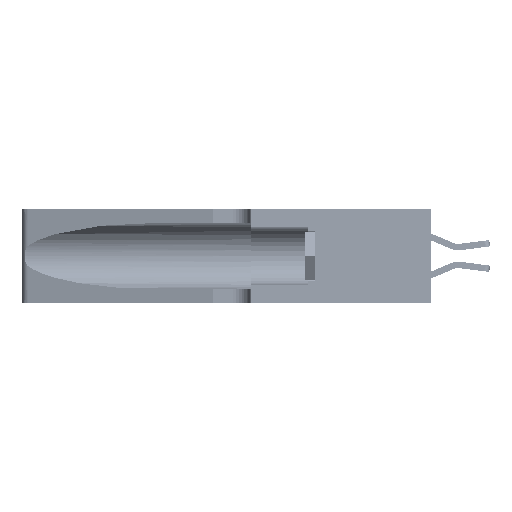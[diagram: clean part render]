
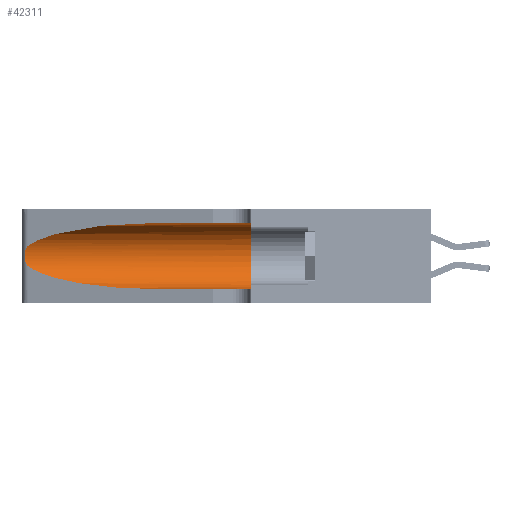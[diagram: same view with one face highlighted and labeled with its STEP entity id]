
A CAD part, left-side view. The second image highlights one B-rep face of the part: STEP entity #42311.
In plain terms, the highlighted cylindrical face has radius 3.308 mm (diameter 6.617 mm), a partial arc.
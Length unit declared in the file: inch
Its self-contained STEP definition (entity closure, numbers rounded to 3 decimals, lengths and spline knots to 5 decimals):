
#1791 = B_SPLINE_CURVE_WITH_KNOTS ( 'NONE', 3,
 ( #13094, #17264, #5121, #40816, #17089, #44774, #29031, #45111, #5292, #5470, #9422, #37172, #38352, #14465 ),
 .UNSPECIFIED., .F., .F.,
 ( 4, 2, 2, 2, 2, 2, 4 ),
 ( 0., 0.00027, 0.00053, 0.00107, 0.0016, 0.00187, 0.00214 ),
 .UNSPECIFIED. ) ;
#2441 = EDGE_CURVE ( 'NONE', #7598, #33572, #5179, .T. ) ;
#2473 = ORIENTED_EDGE ( 'NONE', *, *, #24177, .T. ) ;
#4819 = CARTESIAN_POINT ( 'NONE',  ( 0.18966, 0.96281, 0.31525 ) ) ;
#4823 = CARTESIAN_POINT ( 'NONE',  ( 0.1305, 0.35, 0.185 ) ) ;
#5121 = CARTESIAN_POINT ( 'NONE',  ( 0.25639, 1.23184, 0.21858 ) ) ;
#5179 = CIRCLE ( 'NONE', #12178, 0.13025 ) ;
#5292 = CARTESIAN_POINT ( 'NONE',  ( 0.26017, 1.23833, 0.17102 ) ) ;
#5470 = CARTESIAN_POINT ( 'NONE',  ( 0.25856, 1.23593, 0.16098 ) ) ;
#7160 = ORIENTED_EDGE ( 'NONE', *, *, #2441, .F. ) ;
#7336 = EDGE_LOOP ( 'NONE', ( #2473, #26420, #42686, #13716, #7160, #28904 ) ) ;
#7598 = VERTEX_POINT ( 'NONE', #31393 ) ;
#7652 = CARTESIAN_POINT ( 'NONE',  ( 0.1305, 0.72297, 0.05475 ) ) ;
#8062 = CARTESIAN_POINT ( 'NONE',  ( 0.25487, 1.22718, 0.14631 ) ) ;
#8088 = CARTESIAN_POINT ( 'NONE',  ( 0.1305, 1.61858, 0.05475 ) ) ;
#9422 = CARTESIAN_POINT ( 'NONE',  ( 0.25789, 1.23486, 0.15765 ) ) ;
#9852 = CARTESIAN_POINT ( 'NONE',  ( 0.1305, 0.35, 0.05475 ) ) ;
#10421 = VECTOR ( 'NONE', #28705, 39.37008 ) ;
#12178 = AXIS2_PLACEMENT_3D ( 'NONE', #4823, #48084, #44299 ) ;
#12336 = CARTESIAN_POINT ( 'NONE',  ( 0.1305, 0.72297, 0.31525 ) ) ;
#12973 = CARTESIAN_POINT ( 'NONE',  ( 0.1305, 0.72297, 0.31525 ) ) ;
#13094 = CARTESIAN_POINT ( 'NONE',  ( 0.25487, 1.22718, 0.22369 ) ) ;
#13452 = CARTESIAN_POINT ( 'NONE',  ( 0.1305, 1.61858, 0.31525 ) ) ;
#13587 = AXIS2_PLACEMENT_3D ( 'NONE', #41550, #18192, #29796 ) ;
#13644 = EDGE_CURVE ( 'NONE', #45733, #33572, #19347, .T. ) ;
#13716 = ORIENTED_EDGE ( 'NONE', *, *, #13644, .T. ) ;
#14093 = CYLINDRICAL_SURFACE ( 'NONE', #13587, 0.13025 ) ;
#14465 = CARTESIAN_POINT ( 'NONE',  ( 0.25487, 1.22718, 0.14631 ) ) ;
#15730 = EDGE_CURVE ( 'NONE', #23442, #7598, #46346, .T. ) ;
#17089 = CARTESIAN_POINT ( 'NONE',  ( 0.25854, 1.2359, 0.20912 ) ) ;
#17264 = CARTESIAN_POINT ( 'NONE',  ( 0.25555, 1.22994, 0.2215 ) ) ;
#18192 = DIRECTION ( 'NONE',  ( 0., -1., 0. ) ) ;
#18900 = VERTEX_POINT ( 'NONE', #8062 ) ;
#19347 = LINE ( 'NONE', #8088, #29872 ) ;
#23433 = FACE_OUTER_BOUND ( 'NONE', #7336, .T. ) ;
#23442 = VERTEX_POINT ( 'NONE', #12336 ) ;
#24177 = EDGE_CURVE ( 'NONE', #23442, #38412, #40849, .T. ) ;
#24228 = CARTESIAN_POINT ( 'NONE',  ( 0.25487, 1.22718, 0.14631 ) ) ;
#24460 = CARTESIAN_POINT ( 'NONE',  ( 0.2373, 1.15595, 0.28018 ) ) ;
#26420 = ORIENTED_EDGE ( 'NONE', *, *, #30126, .T. ) ;
#28477 = CARTESIAN_POINT ( 'NONE',  ( 0.2373, 1.15595, 0.08982 ) ) ;
#28705 = DIRECTION ( 'NONE',  ( 0., -1., 0. ) ) ;
#28904 = ORIENTED_EDGE ( 'NONE', *, *, #15730, .F. ) ;
#29031 = CARTESIAN_POINT ( 'NONE',  ( 0.26075, 1.23896, 0.19203 ) ) ;
#29796 = DIRECTION ( 'NONE',  ( 0., 0., -1. ) ) ;
#29872 = VECTOR ( 'NONE', #43427, 39.37008 ) ;
#30126 = EDGE_CURVE ( 'NONE', #38412, #18900, #1791, .T. ) ;
#31393 = CARTESIAN_POINT ( 'NONE',  ( 0.1305, 0.35, 0.31525 ) ) ;
#32287 = CARTESIAN_POINT ( 'NONE',  ( 0.18966, 0.96281, 0.05475 ) ) ;
#32525 = CARTESIAN_POINT ( 'NONE',  ( 0.25487, 1.22718, 0.22369 ) ) ;
#33572 = VERTEX_POINT ( 'NONE', #9852 ) ;
#37172 = CARTESIAN_POINT ( 'NONE',  ( 0.25639, 1.23186, 0.15144 ) ) ;
#38352 = CARTESIAN_POINT ( 'NONE',  ( 0.25555, 1.22993, 0.14849 ) ) ;
#38412 = VERTEX_POINT ( 'NONE', #43135 ) ;
#40816 = CARTESIAN_POINT ( 'NONE',  ( 0.25787, 1.23484, 0.2124 ) ) ;
#40849 =( BOUNDED_CURVE ( )  B_SPLINE_CURVE ( 3, ( #12973, #4819, #24460, #32525 ),
 .UNSPECIFIED., .F., .T. ) 
 B_SPLINE_CURVE_WITH_KNOTS ( ( 4, 4 ),
 ( 1.5708, 2.84003 ),
 .UNSPECIFIED. ) 
 CURVE ( )  GEOMETRIC_REPRESENTATION_ITEM ( )  RATIONAL_B_SPLINE_CURVE ( ( 1., 0.87, 0.87, 1. ) ) 
 REPRESENTATION_ITEM ( '' )  );
#41347 = EDGE_CURVE ( 'NONE', #18900, #45733, #49977, .T. ) ;
#41550 = CARTESIAN_POINT ( 'NONE',  ( 0.1305, 1.61858, 0.185 ) ) ;
#42311 = ADVANCED_FACE ( 'NONE', ( #23433 ), #14093, .F. ) ;
#42686 = ORIENTED_EDGE ( 'NONE', *, *, #41347, .T. ) ;
#43135 = CARTESIAN_POINT ( 'NONE',  ( 0.25487, 1.22718, 0.22369 ) ) ;
#43427 = DIRECTION ( 'NONE',  ( 0., -1., 0. ) ) ;
#44299 = DIRECTION ( 'NONE',  ( 0., 0., 1. ) ) ;
#44774 = CARTESIAN_POINT ( 'NONE',  ( 0.26018, 1.23835, 0.19895 ) ) ;
#45111 = CARTESIAN_POINT ( 'NONE',  ( 0.26075, 1.23896, 0.178 ) ) ;
#45733 = VERTEX_POINT ( 'NONE', #7652 ) ;
#46346 = LINE ( 'NONE', #13452, #10421 ) ;
#48012 = CARTESIAN_POINT ( 'NONE',  ( 0.1305, 0.72297, 0.05475 ) ) ;
#48084 = DIRECTION ( 'NONE',  ( 0., 1., 0. ) ) ;
#49977 =( BOUNDED_CURVE ( )  B_SPLINE_CURVE ( 3, ( #24228, #28477, #32287, #48012 ),
 .UNSPECIFIED., .F., .F. ) 
 B_SPLINE_CURVE_WITH_KNOTS ( ( 4, 4 ),
 ( 3.44316, 4.71239 ),
 .UNSPECIFIED. ) 
 CURVE ( )  GEOMETRIC_REPRESENTATION_ITEM ( )  RATIONAL_B_SPLINE_CURVE ( ( 1., 0.87, 0.87, 1. ) ) 
 REPRESENTATION_ITEM ( '' )  );
